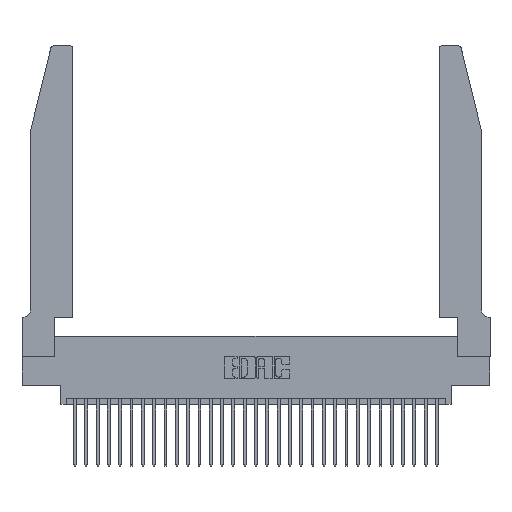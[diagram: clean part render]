
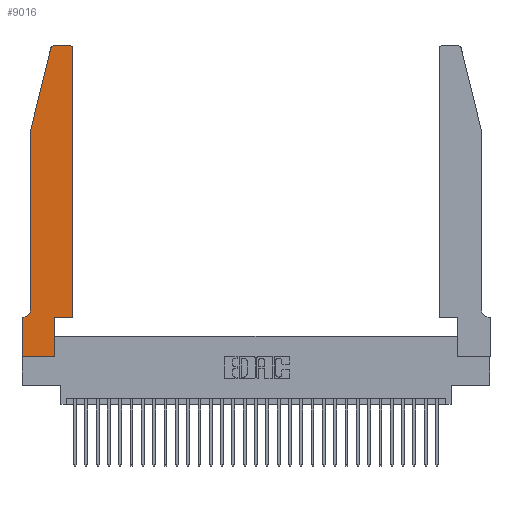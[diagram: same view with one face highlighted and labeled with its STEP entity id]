
A CAD part, top view. The second image highlights one B-rep face of the part: STEP entity #9016.
In plain terms, the highlighted planar face has unit normal (0, 0, 1).
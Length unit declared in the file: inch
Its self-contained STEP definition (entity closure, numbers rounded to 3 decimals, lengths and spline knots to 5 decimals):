
#285 = ORIENTED_EDGE ( 'NONE', *, *, #27086, .T. ) ;
#510 = CARTESIAN_POINT ( 'NONE',  ( 0.0055, 0.42, 0.37 ) ) ;
#592 = EDGE_CURVE ( 'NONE', #14423, #19716, #30358, .T. ) ;
#1482 = DIRECTION ( 'NONE',  ( 0., 1., 0. ) ) ;
#3070 = DIRECTION ( 'NONE',  ( -1., 0., 0. ) ) ;
#3108 = EDGE_CURVE ( 'NONE', #6799, #14423, #30791, .T. ) ;
#3182 = CARTESIAN_POINT ( 'NONE',  ( 0.0755, 0.35, 0.37 ) ) ;
#4431 = EDGE_CURVE ( 'NONE', #6984, #23497, #27303, .T. ) ;
#4503 = CARTESIAN_POINT ( 'NONE',  ( 0.0755, 0.42, 0.37 ) ) ;
#4592 = DIRECTION ( 'NONE',  ( 0., 1., 0. ) ) ;
#4797 = AXIS2_PLACEMENT_3D ( 'NONE', #510, #17977, #3070 ) ;
#4909 = ORIENTED_EDGE ( 'NONE', *, *, #4431, .T. ) ;
#5462 = PLANE ( 'NONE',  #9109 ) ;
#5663 = VERTEX_POINT ( 'NONE', #4503 ) ;
#5763 = EDGE_LOOP ( 'NONE', ( #12296, #12081, #26083, #21312, #24219, #285, #4909, #10100, #18606, #28627, #16847, #20418 ) ) ;
#6342 = EDGE_CURVE ( 'NONE', #19716, #20712, #30589, .T. ) ;
#6522 = FACE_OUTER_BOUND ( 'NONE', #5763, .T. ) ;
#6799 = VERTEX_POINT ( 'NONE', #13675 ) ;
#6984 = VERTEX_POINT ( 'NONE', #31531 ) ;
#7010 = DIRECTION ( 'NONE',  ( 0., -1., 0. ) ) ;
#7162 = CARTESIAN_POINT ( 'NONE',  ( 0., 0., 0.37 ) ) ;
#7526 = EDGE_CURVE ( 'NONE', #20889, #8452, #25888, .T. ) ;
#7778 = VECTOR ( 'NONE', #28642, 39.37008 ) ;
#8216 = CIRCLE ( 'NONE', #21483, 0.03 ) ;
#8452 = VERTEX_POINT ( 'NONE', #27937 ) ;
#8778 = EDGE_CURVE ( 'NONE', #20712, #5663, #18577, .T. ) ;
#9016 = ADVANCED_FACE ( 'NONE', ( #6522 ), #5462, .T. ) ;
#9109 = AXIS2_PLACEMENT_3D ( 'NONE', #22893, #25352, #10614 ) ;
#9698 = DIRECTION ( 'NONE',  ( 0., -1., 0. ) ) ;
#10100 = ORIENTED_EDGE ( 'NONE', *, *, #11191, .T. ) ;
#10612 = CARTESIAN_POINT ( 'NONE',  ( 0.25487, 2.72718, 0.37 ) ) ;
#10614 = DIRECTION ( 'NONE',  ( 1., 0., 0. ) ) ;
#10767 = DIRECTION ( 'NONE',  ( 0., 0., 1. ) ) ;
#11086 = VECTOR ( 'NONE', #15485, 39.37008 ) ;
#11191 = EDGE_CURVE ( 'NONE', #23497, #29922, #24207, .T. ) ;
#12081 = ORIENTED_EDGE ( 'NONE', *, *, #592, .T. ) ;
#12296 = ORIENTED_EDGE ( 'NONE', *, *, #3108, .T. ) ;
#12783 = CARTESIAN_POINT ( 'NONE',  ( 0.2865, 0.35, 0.37 ) ) ;
#12810 = VECTOR ( 'NONE', #7010, 39.37008 ) ;
#13193 = DIRECTION ( 'NONE',  ( 0., 0., 1. ) ) ;
#13198 = CARTESIAN_POINT ( 'NONE',  ( 0.284, 2.72, 0.37 ) ) ;
#13254 = CIRCLE ( 'NONE', #4797, 0.07 ) ;
#13470 = EDGE_CURVE ( 'NONE', #5663, #27298, #13254, .T. ) ;
#13605 = VECTOR ( 'NONE', #1482, 39.37008 ) ;
#13675 = CARTESIAN_POINT ( 'NONE',  ( 0.4205, 2.75, 0.37 ) ) ;
#14368 = VECTOR ( 'NONE', #27922, 39.37008 ) ;
#14389 = LINE ( 'NONE', #23753, #13605 ) ;
#14423 = VERTEX_POINT ( 'NONE', #21480 ) ;
#14687 = DIRECTION ( 'NONE',  ( -0.239, -0.971, 0. ) ) ;
#15149 = LINE ( 'NONE', #3182, #14368 ) ;
#15485 = DIRECTION ( 'NONE',  ( 1., 0., 0. ) ) ;
#16847 = ORIENTED_EDGE ( 'NONE', *, *, #7526, .T. ) ;
#17603 = VECTOR ( 'NONE', #14687, 39.37008 ) ;
#17977 = DIRECTION ( 'NONE',  ( 0., 0., -1. ) ) ;
#18577 = LINE ( 'NONE', #29205, #12810 ) ;
#18606 = ORIENTED_EDGE ( 'NONE', *, *, #19869, .T. ) ;
#19085 = EDGE_CURVE ( 'NONE', #8452, #6799, #8216, .T. ) ;
#19104 = CARTESIAN_POINT ( 'NONE',  ( 0.4505, 0.35, 0.37 ) ) ;
#19238 = VECTOR ( 'NONE', #9698, 39.37008 ) ;
#19301 = DIRECTION ( 'NONE',  ( -1., 0., 0. ) ) ;
#19716 = VERTEX_POINT ( 'NONE', #10612 ) ;
#19862 = EDGE_CURVE ( 'NONE', #24590, #20889, #20940, .T. ) ;
#19869 = EDGE_CURVE ( 'NONE', #29922, #24590, #14389, .T. ) ;
#20184 = VECTOR ( 'NONE', #4592, 39.37008 ) ;
#20418 = ORIENTED_EDGE ( 'NONE', *, *, #19085, .T. ) ;
#20712 = VERTEX_POINT ( 'NONE', #29247 ) ;
#20889 = VERTEX_POINT ( 'NONE', #25097 ) ;
#20940 = LINE ( 'NONE', #21179, #7778 ) ;
#21179 = CARTESIAN_POINT ( 'NONE',  ( 0.4505, 0.35, 0.37 ) ) ;
#21312 = ORIENTED_EDGE ( 'NONE', *, *, #8778, .T. ) ;
#21480 = CARTESIAN_POINT ( 'NONE',  ( 0.284, 2.75, 0.37 ) ) ;
#21483 = AXIS2_PLACEMENT_3D ( 'NONE', #25486, #10767, #27932 ) ;
#21792 = AXIS2_PLACEMENT_3D ( 'NONE', #13198, #13193, #23120 ) ;
#22893 = CARTESIAN_POINT ( 'NONE',  ( 0., 0.35, 0.37 ) ) ;
#22958 = CARTESIAN_POINT ( 'NONE',  ( 0., 0., 0.37 ) ) ;
#23120 = DIRECTION ( 'NONE',  ( 1., 0., 0. ) ) ;
#23497 = VERTEX_POINT ( 'NONE', #22958 ) ;
#23563 = VECTOR ( 'NONE', #19301, 39.37008 ) ;
#23753 = CARTESIAN_POINT ( 'NONE',  ( 0.2865, 0.35, 0.37 ) ) ;
#24207 = LINE ( 'NONE', #25250, #11086 ) ;
#24219 = ORIENTED_EDGE ( 'NONE', *, *, #13470, .T. ) ;
#24471 = CARTESIAN_POINT ( 'NONE',  ( 0.0755, 2., 0.37 ) ) ;
#24590 = VERTEX_POINT ( 'NONE', #12783 ) ;
#25097 = CARTESIAN_POINT ( 'NONE',  ( 0.4505, 0.35, 0.37 ) ) ;
#25250 = CARTESIAN_POINT ( 'NONE',  ( 0., 0., 0.37 ) ) ;
#25352 = DIRECTION ( 'NONE',  ( 0., 0., 1. ) ) ;
#25486 = CARTESIAN_POINT ( 'NONE',  ( 0.4205, 2.72, 0.37 ) ) ;
#25888 = LINE ( 'NONE', #19104, #20184 ) ;
#26083 = ORIENTED_EDGE ( 'NONE', *, *, #6342, .T. ) ;
#26864 = CARTESIAN_POINT ( 'NONE',  ( 0.2865, 0., 0.37 ) ) ;
#27086 = EDGE_CURVE ( 'NONE', #27298, #6984, #15149, .T. ) ;
#27298 = VERTEX_POINT ( 'NONE', #28443 ) ;
#27303 = LINE ( 'NONE', #7162, #19238 ) ;
#27922 = DIRECTION ( 'NONE',  ( -1., 0., 0. ) ) ;
#27932 = DIRECTION ( 'NONE',  ( 1., 0., 0. ) ) ;
#27937 = CARTESIAN_POINT ( 'NONE',  ( 0.4505, 2.72, 0.37 ) ) ;
#28443 = CARTESIAN_POINT ( 'NONE',  ( 0.0055, 0.35, 0.37 ) ) ;
#28627 = ORIENTED_EDGE ( 'NONE', *, *, #19862, .T. ) ;
#28642 = DIRECTION ( 'NONE',  ( 1., 0., 0. ) ) ;
#29205 = CARTESIAN_POINT ( 'NONE',  ( 0.0755, 2., 0.37 ) ) ;
#29247 = CARTESIAN_POINT ( 'NONE',  ( 0.0755, 2., 0.37 ) ) ;
#29922 = VERTEX_POINT ( 'NONE', #26864 ) ;
#30358 = CIRCLE ( 'NONE', #21792, 0.03 ) ;
#30589 = LINE ( 'NONE', #24471, #17603 ) ;
#30791 = LINE ( 'NONE', #31469, #23563 ) ;
#31469 = CARTESIAN_POINT ( 'NONE',  ( 0.2605, 2.75, 0.37 ) ) ;
#31531 = CARTESIAN_POINT ( 'NONE',  ( 0., 0.35, 0.37 ) ) ;
